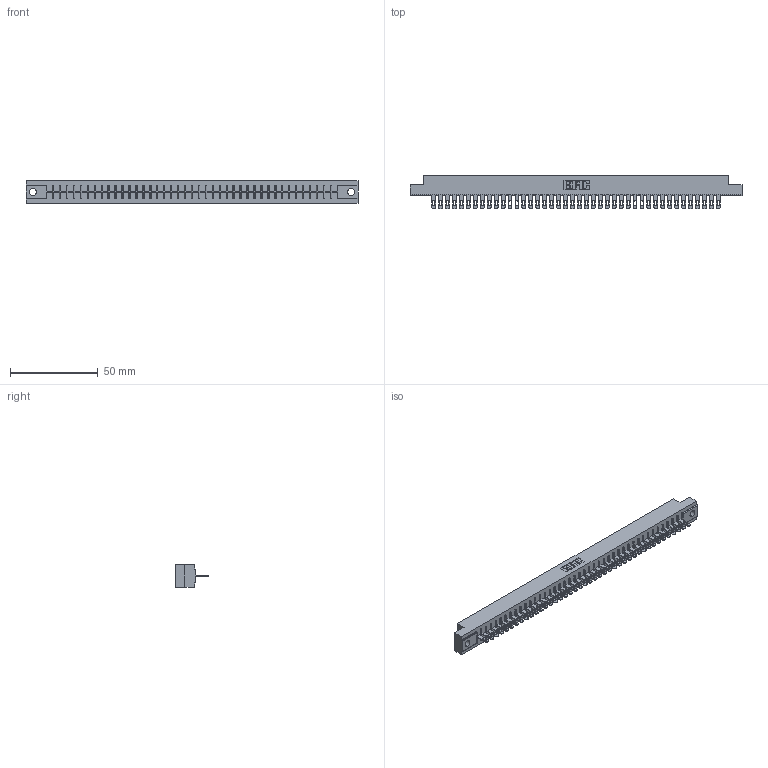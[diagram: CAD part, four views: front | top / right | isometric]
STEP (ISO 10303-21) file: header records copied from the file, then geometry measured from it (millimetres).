
FILE_DESCRIPTION (( 'STEP AP203' ), '1' );
FILE_NAME ('356-042-400-104.STEP', '2020-09-24T01:17:51', ( '' ), ( '' ), 'SwSTEP 2.0', 'SolidWorks 2020', '' );
FILE_SCHEMA (( 'CONFIG_CONTROL_DESIGN' ));
Length unit declared in the file: inch
Products named in the file (3): 306 Part_.156 Dia; 306-290-001_100; 356-042-400-104
Assembly tree (43 placements, depth 2):
  356-042-400-104
    306 Part_.156 Dia
    306-290-001_100  x42
Bounding box: 189.43 x 18.87 x 12.7 mm (x, y, z)
Volume: 20978.6 mm3; surface area: 22091.3 mm2
Topology: 43 solids, 43 shells, 3322 faces, 9382 edges, 6028 vertices
Faces by surface type: plane 2182, cylinder 972, sphere 168
Entity records: 39749 total; most frequent: CARTESIAN_POINT 6679, ORIENTED_EDGE 6620, DIRECTION 6578, EDGE_CURVE 3310, LINE 2596, VECTOR 2596, VERTEX_POINT 2092, AXIS2_PLACEMENT_3D 1991
